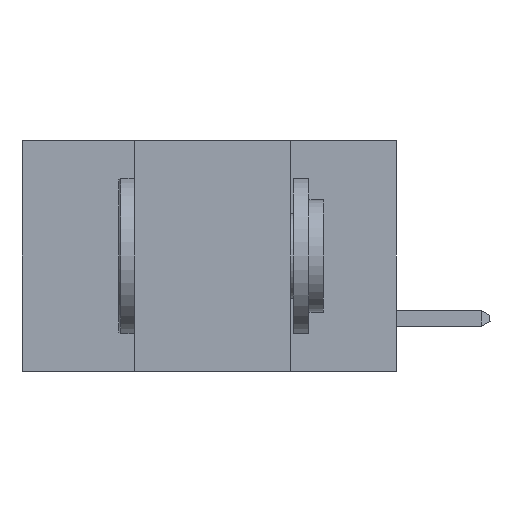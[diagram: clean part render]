
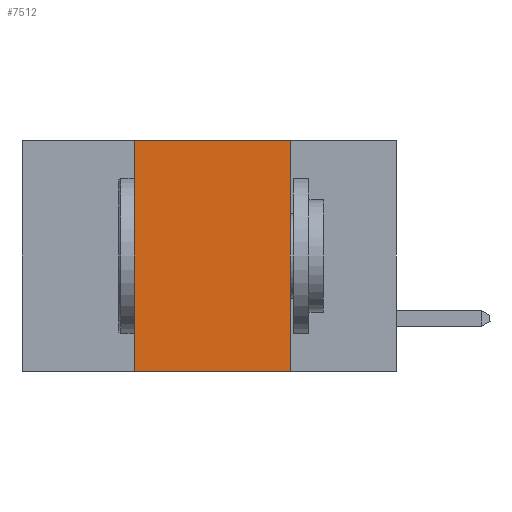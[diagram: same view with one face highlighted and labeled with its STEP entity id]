
A CAD part, left-side view. The second image highlights one B-rep face of the part: STEP entity #7512.
In plain terms, the highlighted planar face has unit normal (-1, 0, 0).
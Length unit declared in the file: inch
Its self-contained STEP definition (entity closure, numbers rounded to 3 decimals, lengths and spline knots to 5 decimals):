
#237 = VERTEX_POINT ( 'NONE', #6185 ) ;
#874 = VECTOR ( 'NONE', #9214, 39.37008 ) ;
#3721 = LINE ( 'NONE', #10590, #27677 ) ;
#5119 = AXIS2_PLACEMENT_3D ( 'NONE', #10954, #10757, #10530 ) ;
#6185 = CARTESIAN_POINT ( 'NONE',  ( 0., 0.17, -0.37 ) ) ;
#7159 = VERTEX_POINT ( 'NONE', #19284 ) ;
#7512 = ADVANCED_FACE ( 'NONE', ( #8747 ), #10876, .F. ) ;
#7982 = DIRECTION ( 'NONE',  ( 0., -1., 0. ) ) ;
#8131 = VECTOR ( 'NONE', #27326, 39.37008 ) ;
#8154 = ORIENTED_EDGE ( 'NONE', *, *, #12265, .F. ) ;
#8747 = FACE_OUTER_BOUND ( 'NONE', #25770, .T. ) ;
#9214 = DIRECTION ( 'NONE',  ( 0., 0., -1. ) ) ;
#9312 = CARTESIAN_POINT ( 'NONE',  ( 0., 0.17, 0. ) ) ;
#10530 = DIRECTION ( 'NONE',  ( 0., 0., -1. ) ) ;
#10590 = CARTESIAN_POINT ( 'NONE',  ( 0., 0.6, 0. ) ) ;
#10757 = DIRECTION ( 'NONE',  ( 1., 0., 0. ) ) ;
#10876 = PLANE ( 'NONE',  #5119 ) ;
#10954 = CARTESIAN_POINT ( 'NONE',  ( 0., 0.6, 0. ) ) ;
#12192 = ORIENTED_EDGE ( 'NONE', *, *, #23801, .F. ) ;
#12265 = EDGE_CURVE ( 'NONE', #19881, #20715, #3721, .T. ) ;
#12989 = VECTOR ( 'NONE', #7982, 39.37008 ) ;
#13592 = LINE ( 'NONE', #9312, #874 ) ;
#14277 = LINE ( 'NONE', #22774, #8131 ) ;
#17643 = ORIENTED_EDGE ( 'NONE', *, *, #22292, .T. ) ;
#19036 = CARTESIAN_POINT ( 'NONE',  ( 0., 0.17, 0. ) ) ;
#19284 = CARTESIAN_POINT ( 'NONE',  ( 0., 0.42, -0.37 ) ) ;
#19881 = VERTEX_POINT ( 'NONE', #23320 ) ;
#20715 = VERTEX_POINT ( 'NONE', #19036 ) ;
#20889 = ORIENTED_EDGE ( 'NONE', *, *, #26840, .F. ) ;
#22292 = EDGE_CURVE ( 'NONE', #7159, #237, #24496, .T. ) ;
#22774 = CARTESIAN_POINT ( 'NONE',  ( 0., 0.42, 0. ) ) ;
#23320 = CARTESIAN_POINT ( 'NONE',  ( 0., 0.42, 0. ) ) ;
#23801 = EDGE_CURVE ( 'NONE', #7159, #19881, #14277, .T. ) ;
#24154 = CARTESIAN_POINT ( 'NONE',  ( 0., 0.6, -0.37 ) ) ;
#24384 = DIRECTION ( 'NONE',  ( 0., -1., 0. ) ) ;
#24496 = LINE ( 'NONE', #24154, #12989 ) ;
#25770 = EDGE_LOOP ( 'NONE', ( #20889, #8154, #12192, #17643 ) ) ;
#26840 = EDGE_CURVE ( 'NONE', #20715, #237, #13592, .T. ) ;
#27326 = DIRECTION ( 'NONE',  ( 0., 0., 1. ) ) ;
#27677 = VECTOR ( 'NONE', #24384, 39.37008 ) ;
